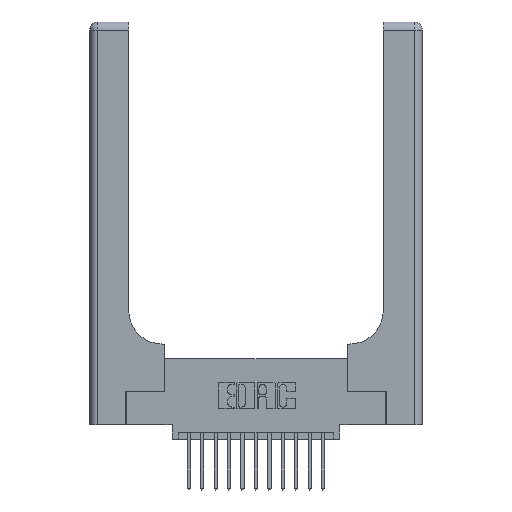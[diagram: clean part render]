
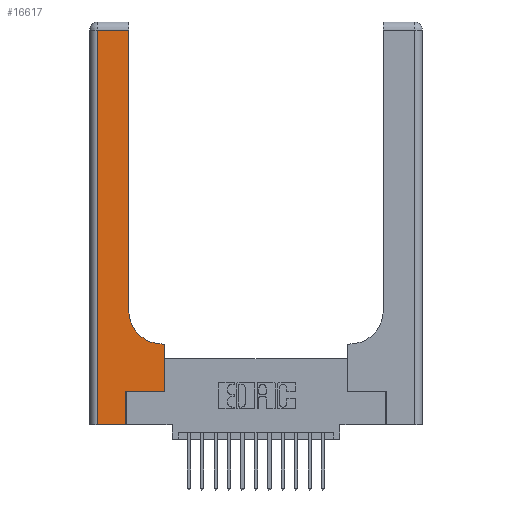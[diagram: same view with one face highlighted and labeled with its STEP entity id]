
A CAD part, top view. The second image highlights one B-rep face of the part: STEP entity #16617.
In plain terms, the highlighted planar face has unit normal (0, 0, 1).
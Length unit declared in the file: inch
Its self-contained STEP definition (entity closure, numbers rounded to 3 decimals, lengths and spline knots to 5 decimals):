
#95 = VECTOR ( 'NONE', #130, 39.37008 ) ;
#130 = DIRECTION ( 'NONE',  ( 1., 0., 0. ) ) ;
#489 = PLANE ( 'NONE',  #18111 ) ;
#1368 = DIRECTION ( 'NONE',  ( 0., 1., 0. ) ) ;
#1432 = ORIENTED_EDGE ( 'NONE', *, *, #4527, .T. ) ;
#1572 = ORIENTED_EDGE ( 'NONE', *, *, #14485, .T. ) ;
#1655 = VECTOR ( 'NONE', #1368, 39.37008 ) ;
#1678 = CARTESIAN_POINT ( 'NONE',  ( 0.269, 0., 0.37 ) ) ;
#1749 = CARTESIAN_POINT ( 'NONE',  ( 0.5415, 0.85, 0.37 ) ) ;
#1772 = CARTESIAN_POINT ( 'NONE',  ( 0.269, 0.25, 0.37 ) ) ;
#1828 = DIRECTION ( 'NONE',  ( 0., -1., 0. ) ) ;
#1863 = CARTESIAN_POINT ( 'NONE',  ( 0., 3., 0.37 ) ) ;
#1888 = VECTOR ( 'NONE', #14742, 39.37008 ) ;
#1931 = DIRECTION ( 'NONE',  ( 0., 0., -1. ) ) ;
#2122 = AXIS2_PLACEMENT_3D ( 'NONE', #1749, #11626, #3177 ) ;
#2141 = ORIENTED_EDGE ( 'NONE', *, *, #9288, .T. ) ;
#2280 = FACE_OUTER_BOUND ( 'NONE', #13041, .T. ) ;
#2333 = LINE ( 'NONE', #6371, #1888 ) ;
#3177 = DIRECTION ( 'NONE',  ( 1., 0., 0. ) ) ;
#3772 = CARTESIAN_POINT ( 'NONE',  ( 0.5585, 0.6, 0.37 ) ) ;
#4237 = DIRECTION ( 'NONE',  ( 0., 1., 0. ) ) ;
#4527 = EDGE_CURVE ( 'NONE', #10470, #6637, #2333, .T. ) ;
#4616 = LINE ( 'NONE', #5658, #15340 ) ;
#4848 = EDGE_CURVE ( 'NONE', #12516, #17528, #16988, .T. ) ;
#5111 = EDGE_CURVE ( 'NONE', #17528, #11053, #6348, .T. ) ;
#5319 = CIRCLE ( 'NONE', #2122, 0.25 ) ;
#5658 = CARTESIAN_POINT ( 'NONE',  ( 0.269, 0., 0.37 ) ) ;
#5918 = VECTOR ( 'NONE', #1828, 39.37008 ) ;
#6000 = CARTESIAN_POINT ( 'NONE',  ( 0.2915, 2.94, 0.37 ) ) ;
#6348 = LINE ( 'NONE', #9073, #9656 ) ;
#6371 = CARTESIAN_POINT ( 'NONE',  ( 0.2915, 0.6, 0.37 ) ) ;
#6512 = VERTEX_POINT ( 'NONE', #6612 ) ;
#6612 = CARTESIAN_POINT ( 'NONE',  ( 0.269, 0.25, 0.37 ) ) ;
#6637 = VERTEX_POINT ( 'NONE', #11021 ) ;
#7143 = ORIENTED_EDGE ( 'NONE', *, *, #4848, .T. ) ;
#7700 = LINE ( 'NONE', #16941, #95 ) ;
#7858 = VERTEX_POINT ( 'NONE', #8264 ) ;
#8264 = CARTESIAN_POINT ( 'NONE',  ( 0.06, 0., 0.37 ) ) ;
#8745 = CARTESIAN_POINT ( 'NONE',  ( 0.2915, 0.85, 0.37 ) ) ;
#8754 = EDGE_CURVE ( 'NONE', #15369, #10470, #16221, .T. ) ;
#9073 = CARTESIAN_POINT ( 'NONE',  ( 0., 2.94, 0.37 ) ) ;
#9288 = EDGE_CURVE ( 'NONE', #6637, #12516, #5319, .T. ) ;
#9656 = VECTOR ( 'NONE', #17332, 39.37008 ) ;
#9681 = LINE ( 'NONE', #14455, #5918 ) ;
#9752 = VECTOR ( 'NONE', #14462, 39.37008 ) ;
#10045 = ORIENTED_EDGE ( 'NONE', *, *, #13679, .T. ) ;
#10470 = VERTEX_POINT ( 'NONE', #3772 ) ;
#11021 = CARTESIAN_POINT ( 'NONE',  ( 0.5415, 0.6, 0.37 ) ) ;
#11053 = VERTEX_POINT ( 'NONE', #17539 ) ;
#11554 = ORIENTED_EDGE ( 'NONE', *, *, #14859, .T. ) ;
#11626 = DIRECTION ( 'NONE',  ( 0., 0., -1. ) ) ;
#11802 = DIRECTION ( 'NONE',  ( -1., 0., 0. ) ) ;
#12516 = VERTEX_POINT ( 'NONE', #8745 ) ;
#12551 = VECTOR ( 'NONE', #16116, 39.37008 ) ;
#12574 = EDGE_CURVE ( 'NONE', #6512, #15369, #13423, .T. ) ;
#12649 = CARTESIAN_POINT ( 'NONE',  ( 0.2915, 3., 0.37 ) ) ;
#13041 = EDGE_LOOP ( 'NONE', ( #7143, #13885, #1572, #11554, #10045, #16543, #15150, #1432, #2141 ) ) ;
#13423 = LINE ( 'NONE', #1772, #9752 ) ;
#13679 = EDGE_CURVE ( 'NONE', #17916, #6512, #4616, .T. ) ;
#13885 = ORIENTED_EDGE ( 'NONE', *, *, #5111, .T. ) ;
#14455 = CARTESIAN_POINT ( 'NONE',  ( 0.06, 3., 0.37 ) ) ;
#14462 = DIRECTION ( 'NONE',  ( 1., 0., 0. ) ) ;
#14485 = EDGE_CURVE ( 'NONE', #11053, #7858, #9681, .T. ) ;
#14742 = DIRECTION ( 'NONE',  ( -1., 0., 0. ) ) ;
#14756 = CARTESIAN_POINT ( 'NONE',  ( 0.5585, 0.25, 0.37 ) ) ;
#14859 = EDGE_CURVE ( 'NONE', #7858, #17916, #7700, .T. ) ;
#15150 = ORIENTED_EDGE ( 'NONE', *, *, #8754, .T. ) ;
#15340 = VECTOR ( 'NONE', #4237, 39.37008 ) ;
#15369 = VERTEX_POINT ( 'NONE', #15535 ) ;
#15535 = CARTESIAN_POINT ( 'NONE',  ( 0.5585, 0.25, 0.37 ) ) ;
#16116 = DIRECTION ( 'NONE',  ( 0., 1., 0. ) ) ;
#16221 = LINE ( 'NONE', #14756, #12551 ) ;
#16543 = ORIENTED_EDGE ( 'NONE', *, *, #12574, .T. ) ;
#16617 = ADVANCED_FACE ( 'NONE', ( #2280 ), #489, .F. ) ;
#16941 = CARTESIAN_POINT ( 'NONE',  ( 0., 0., 0.37 ) ) ;
#16988 = LINE ( 'NONE', #12649, #1655 ) ;
#17332 = DIRECTION ( 'NONE',  ( -1., 0., 0. ) ) ;
#17528 = VERTEX_POINT ( 'NONE', #6000 ) ;
#17539 = CARTESIAN_POINT ( 'NONE',  ( 0.06, 2.94, 0.37 ) ) ;
#17916 = VERTEX_POINT ( 'NONE', #1678 ) ;
#18111 = AXIS2_PLACEMENT_3D ( 'NONE', #1863, #1931, #11802 ) ;
